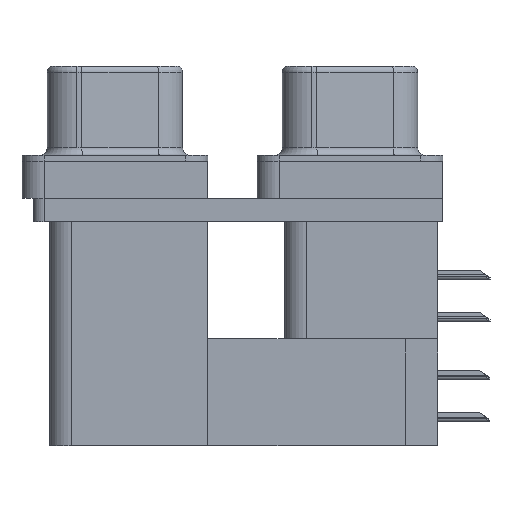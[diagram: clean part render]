
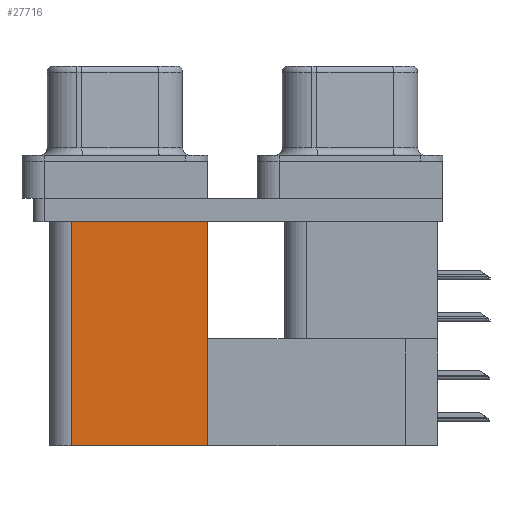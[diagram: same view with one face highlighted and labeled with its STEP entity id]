
A CAD part, left-side view. The second image highlights one B-rep face of the part: STEP entity #27716.
In plain terms, the highlighted planar face has unit normal (-1, 0, 0).
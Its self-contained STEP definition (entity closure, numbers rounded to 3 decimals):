
#44 = DIRECTION ( 'NONE',  ( 0., 0., -1. ) ) ;
#358 = VECTOR ( 'NONE', #39600, 1000. ) ;
#371 = VERTEX_POINT ( 'NONE', #9197 ) ;
#1537 = ORIENTED_EDGE ( 'NONE', *, *, #32665, .F. ) ;
#2913 = ORIENTED_EDGE ( 'NONE', *, *, #5679, .T. ) ;
#4943 = EDGE_LOOP ( 'NONE', ( #25092, #38331, #1537, #2913 ) ) ;
#5679 = EDGE_CURVE ( 'NONE', #371, #13005, #15151, .T. ) ;
#5874 = CARTESIAN_POINT ( 'NONE',  ( 3.7, 9.6, -2.5 ) ) ;
#6274 = LINE ( 'NONE', #5874, #18006 ) ;
#6297 = DIRECTION ( 'NONE',  ( 1., 0., 0. ) ) ;
#6347 = AXIS2_PLACEMENT_3D ( 'NONE', #21037, #6297, #44 ) ;
#6685 = CARTESIAN_POINT ( 'NONE',  ( 3.7, 18.8, -19.2 ) ) ;
#6905 = EDGE_CURVE ( 'NONE', #29692, #24203, #9488, .T. ) ;
#6911 = EDGE_CURVE ( 'NONE', #13005, #24203, #6274, .T. ) ;
#7040 = VECTOR ( 'NONE', #15550, 1000. ) ;
#8344 = LINE ( 'NONE', #14396, #15050 ) ;
#9197 = CARTESIAN_POINT ( 'NONE',  ( 3.7, 9.6, -19.2 ) ) ;
#9488 = LINE ( 'NONE', #34141, #7040 ) ;
#13005 = VERTEX_POINT ( 'NONE', #21010 ) ;
#14396 = CARTESIAN_POINT ( 'NONE',  ( 3.7, 9.6, -19.2 ) ) ;
#14448 = CARTESIAN_POINT ( 'NONE',  ( 3.7, 18.8, -2.5 ) ) ;
#15050 = VECTOR ( 'NONE', #20663, 1000. ) ;
#15151 = LINE ( 'NONE', #21006, #358 ) ;
#15550 = DIRECTION ( 'NONE',  ( 0., 0., 1. ) ) ;
#18006 = VECTOR ( 'NONE', #37169, 1000. ) ;
#18406 = FACE_OUTER_BOUND ( 'NONE', #4943, .T. ) ;
#20663 = DIRECTION ( 'NONE',  ( 0., 1., 0. ) ) ;
#21006 = CARTESIAN_POINT ( 'NONE',  ( 3.7, 9.6, -19.2 ) ) ;
#21010 = CARTESIAN_POINT ( 'NONE',  ( 3.7, 9.6, -2.5 ) ) ;
#21037 = CARTESIAN_POINT ( 'NONE',  ( 3.7, 9.6, -19.2 ) ) ;
#24203 = VERTEX_POINT ( 'NONE', #14448 ) ;
#25092 = ORIENTED_EDGE ( 'NONE', *, *, #6911, .T. ) ;
#27716 = ADVANCED_FACE ( 'NONE', ( #18406 ), #39838, .F. ) ;
#29692 = VERTEX_POINT ( 'NONE', #6685 ) ;
#32665 = EDGE_CURVE ( 'NONE', #371, #29692, #8344, .T. ) ;
#34141 = CARTESIAN_POINT ( 'NONE',  ( 3.7, 18.8, -19.2 ) ) ;
#37169 = DIRECTION ( 'NONE',  ( 0., 1., 0. ) ) ;
#38331 = ORIENTED_EDGE ( 'NONE', *, *, #6905, .F. ) ;
#39600 = DIRECTION ( 'NONE',  ( 0., 0., 1. ) ) ;
#39838 = PLANE ( 'NONE',  #6347 ) ;
